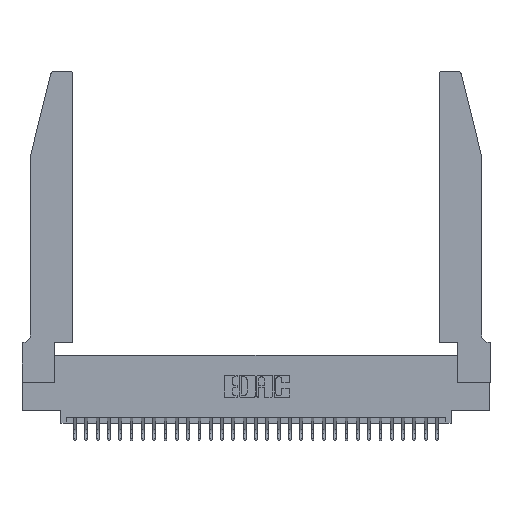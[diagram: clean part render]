
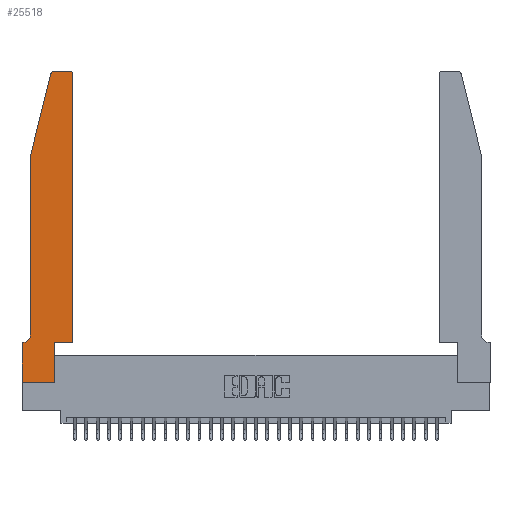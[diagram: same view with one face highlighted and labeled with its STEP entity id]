
A CAD part, top view. The second image highlights one B-rep face of the part: STEP entity #25518.
In plain terms, the highlighted planar face has unit normal (0, 0, 1).
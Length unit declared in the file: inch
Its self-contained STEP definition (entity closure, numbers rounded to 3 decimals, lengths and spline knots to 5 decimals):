
#969 = DIRECTION ( 'NONE',  ( 0., 1., 0. ) ) ;
#1226 = LINE ( 'NONE', #4962, #24919 ) ;
#1673 = VERTEX_POINT ( 'NONE', #25980 ) ;
#2167 = ORIENTED_EDGE ( 'NONE', *, *, #27044, .T. ) ;
#2762 = DIRECTION ( 'NONE',  ( 1., 0., 0. ) ) ;
#3284 = EDGE_CURVE ( 'NONE', #30561, #24411, #25291, .T. ) ;
#3343 = VECTOR ( 'NONE', #12477, 39.37008 ) ;
#3395 = ORIENTED_EDGE ( 'NONE', *, *, #17858, .T. ) ;
#3416 = DIRECTION ( 'NONE',  ( -1., 0., 0. ) ) ;
#4038 = CARTESIAN_POINT ( 'NONE',  ( 0., 0., 0.37 ) ) ;
#4192 = DIRECTION ( 'NONE',  ( 0., 0., 1. ) ) ;
#4202 = VERTEX_POINT ( 'NONE', #20170 ) ;
#4466 = DIRECTION ( 'NONE',  ( -1., 0., 0. ) ) ;
#4962 = CARTESIAN_POINT ( 'NONE',  ( 0.0755, 2., 0.37 ) ) ;
#5196 = CARTESIAN_POINT ( 'NONE',  ( 0.0055, 0.42, 0.37 ) ) ;
#5263 = DIRECTION ( 'NONE',  ( 0., 0., 1. ) ) ;
#5557 = ORIENTED_EDGE ( 'NONE', *, *, #7034, .T. ) ;
#5787 = EDGE_LOOP ( 'NONE', ( #15844, #25480, #2167, #5557, #11977, #26623, #3395, #10581, #31466, #30911, #6289, #23910 ) ) ;
#6289 = ORIENTED_EDGE ( 'NONE', *, *, #23488, .T. ) ;
#7034 = EDGE_CURVE ( 'NONE', #4202, #25654, #1226, .T. ) ;
#7890 = VECTOR ( 'NONE', #15688, 39.37008 ) ;
#8612 = CARTESIAN_POINT ( 'NONE',  ( 0.2865, 0.35, 0.37 ) ) ;
#8691 = VERTEX_POINT ( 'NONE', #17527 ) ;
#9709 = LINE ( 'NONE', #30693, #24067 ) ;
#9955 = LINE ( 'NONE', #19516, #3343 ) ;
#10113 = VERTEX_POINT ( 'NONE', #20284 ) ;
#10260 = CARTESIAN_POINT ( 'NONE',  ( 0.4205, 2.72, 0.37 ) ) ;
#10457 = CARTESIAN_POINT ( 'NONE',  ( 0.0755, 0.42, 0.37 ) ) ;
#10581 = ORIENTED_EDGE ( 'NONE', *, *, #23202, .T. ) ;
#10593 = CARTESIAN_POINT ( 'NONE',  ( 0.2605, 2.75, 0.37 ) ) ;
#10948 = EDGE_CURVE ( 'NONE', #25654, #10113, #23504, .T. ) ;
#11977 = ORIENTED_EDGE ( 'NONE', *, *, #10948, .T. ) ;
#12477 = DIRECTION ( 'NONE',  ( 0., 1., 0. ) ) ;
#12549 = AXIS2_PLACEMENT_3D ( 'NONE', #5196, #22539, #27524 ) ;
#13692 = CARTESIAN_POINT ( 'NONE',  ( 0.4505, 0.35, 0.37 ) ) ;
#13860 = DIRECTION ( 'NONE',  ( 1., 0., 0. ) ) ;
#14087 = VERTEX_POINT ( 'NONE', #22086 ) ;
#14205 = CIRCLE ( 'NONE', #24362, 0.03 ) ;
#14544 = DIRECTION ( 'NONE',  ( 1., 0., 0. ) ) ;
#14632 = VECTOR ( 'NONE', #14544, 39.37008 ) ;
#15688 = DIRECTION ( 'NONE',  ( -0.239, -0.971, 0. ) ) ;
#15779 = LINE ( 'NONE', #4038, #14632 ) ;
#15844 = ORIENTED_EDGE ( 'NONE', *, *, #3284, .T. ) ;
#16440 = DIRECTION ( 'NONE',  ( 1., 0., 0. ) ) ;
#16772 = VECTOR ( 'NONE', #31338, 39.37008 ) ;
#17130 = VECTOR ( 'NONE', #3416, 39.37008 ) ;
#17527 = CARTESIAN_POINT ( 'NONE',  ( 0.2865, 0.35, 0.37 ) ) ;
#17855 = DIRECTION ( 'NONE',  ( 0., -1., 0. ) ) ;
#17858 = EDGE_CURVE ( 'NONE', #20637, #28109, #9709, .T. ) ;
#18551 = AXIS2_PLACEMENT_3D ( 'NONE', #10260, #5263, #2762 ) ;
#18725 = CARTESIAN_POINT ( 'NONE',  ( 0., 0.35, 0.37 ) ) ;
#18729 = LINE ( 'NONE', #22838, #7890 ) ;
#19036 = CARTESIAN_POINT ( 'NONE',  ( 0., 0.35, 0.37 ) ) ;
#19192 = FACE_OUTER_BOUND ( 'NONE', #5787, .T. ) ;
#19262 = EDGE_CURVE ( 'NONE', #8691, #21931, #29585, .T. ) ;
#19516 = CARTESIAN_POINT ( 'NONE',  ( 0.4505, 0.35, 0.37 ) ) ;
#20170 = CARTESIAN_POINT ( 'NONE',  ( 0.0755, 2., 0.37 ) ) ;
#20284 = CARTESIAN_POINT ( 'NONE',  ( 0.0055, 0.35, 0.37 ) ) ;
#20637 = VERTEX_POINT ( 'NONE', #18725 ) ;
#21062 = CARTESIAN_POINT ( 'NONE',  ( 0.4205, 2.75, 0.37 ) ) ;
#21140 = EDGE_CURVE ( 'NONE', #1673, #30561, #26009, .T. ) ;
#21389 = VECTOR ( 'NONE', #4466, 39.37008 ) ;
#21505 = VECTOR ( 'NONE', #969, 39.37008 ) ;
#21931 = VERTEX_POINT ( 'NONE', #13692 ) ;
#22086 = CARTESIAN_POINT ( 'NONE',  ( 0.25487, 2.72718, 0.37 ) ) ;
#22539 = DIRECTION ( 'NONE',  ( 0., 0., -1. ) ) ;
#22838 = CARTESIAN_POINT ( 'NONE',  ( 0.0755, 2., 0.37 ) ) ;
#23202 = EDGE_CURVE ( 'NONE', #28109, #28125, #15779, .T. ) ;
#23231 = AXIS2_PLACEMENT_3D ( 'NONE', #19036, #4192, #13860 ) ;
#23488 = EDGE_CURVE ( 'NONE', #21931, #1673, #9955, .T. ) ;
#23504 = CIRCLE ( 'NONE', #12549, 0.07 ) ;
#23910 = ORIENTED_EDGE ( 'NONE', *, *, #21140, .T. ) ;
#24067 = VECTOR ( 'NONE', #17855, 39.37008 ) ;
#24362 = AXIS2_PLACEMENT_3D ( 'NONE', #26723, #31544, #16440 ) ;
#24411 = VERTEX_POINT ( 'NONE', #28471 ) ;
#24516 = CARTESIAN_POINT ( 'NONE',  ( 0.0755, 0.35, 0.37 ) ) ;
#24919 = VECTOR ( 'NONE', #27947, 39.37008 ) ;
#24952 = EDGE_CURVE ( 'NONE', #28125, #8691, #30520, .T. ) ;
#25291 = LINE ( 'NONE', #10593, #17130 ) ;
#25480 = ORIENTED_EDGE ( 'NONE', *, *, #31784, .T. ) ;
#25518 = ADVANCED_FACE ( 'NONE', ( #19192 ), #31553, .T. ) ;
#25654 = VERTEX_POINT ( 'NONE', #10457 ) ;
#25980 = CARTESIAN_POINT ( 'NONE',  ( 0.4505, 2.72, 0.37 ) ) ;
#26009 = CIRCLE ( 'NONE', #18551, 0.03 ) ;
#26623 = ORIENTED_EDGE ( 'NONE', *, *, #28378, .T. ) ;
#26723 = CARTESIAN_POINT ( 'NONE',  ( 0.284, 2.72, 0.37 ) ) ;
#26896 = CARTESIAN_POINT ( 'NONE',  ( 0., 0., 0.37 ) ) ;
#27044 = EDGE_CURVE ( 'NONE', #14087, #4202, #18729, .T. ) ;
#27111 = CARTESIAN_POINT ( 'NONE',  ( 0.2865, 0., 0.37 ) ) ;
#27524 = DIRECTION ( 'NONE',  ( -1., 0., 0. ) ) ;
#27947 = DIRECTION ( 'NONE',  ( 0., -1., 0. ) ) ;
#27983 = LINE ( 'NONE', #24516, #21389 ) ;
#28109 = VERTEX_POINT ( 'NONE', #26896 ) ;
#28125 = VERTEX_POINT ( 'NONE', #27111 ) ;
#28378 = EDGE_CURVE ( 'NONE', #10113, #20637, #27983, .T. ) ;
#28471 = CARTESIAN_POINT ( 'NONE',  ( 0.284, 2.75, 0.37 ) ) ;
#29585 = LINE ( 'NONE', #31444, #16772 ) ;
#30520 = LINE ( 'NONE', #8612, #21505 ) ;
#30561 = VERTEX_POINT ( 'NONE', #21062 ) ;
#30693 = CARTESIAN_POINT ( 'NONE',  ( 0., 0., 0.37 ) ) ;
#30911 = ORIENTED_EDGE ( 'NONE', *, *, #19262, .T. ) ;
#31338 = DIRECTION ( 'NONE',  ( 1., 0., 0. ) ) ;
#31444 = CARTESIAN_POINT ( 'NONE',  ( 0.4505, 0.35, 0.37 ) ) ;
#31466 = ORIENTED_EDGE ( 'NONE', *, *, #24952, .T. ) ;
#31544 = DIRECTION ( 'NONE',  ( 0., 0., 1. ) ) ;
#31553 = PLANE ( 'NONE',  #23231 ) ;
#31784 = EDGE_CURVE ( 'NONE', #24411, #14087, #14205, .T. ) ;
